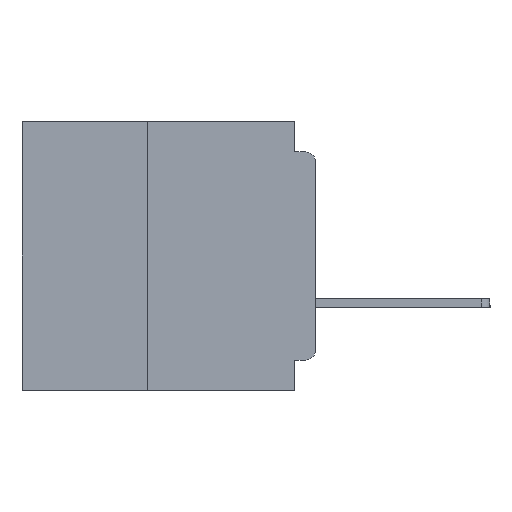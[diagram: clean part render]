
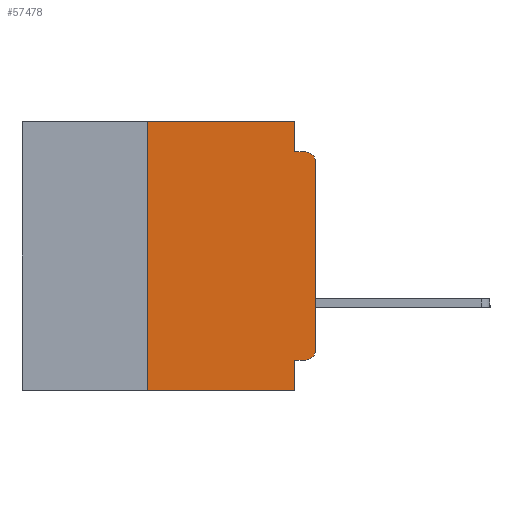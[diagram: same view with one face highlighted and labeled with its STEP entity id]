
A CAD part, left-side view. The second image highlights one B-rep face of the part: STEP entity #57478.
In plain terms, the highlighted planar face has unit normal (-1, 0, 0).
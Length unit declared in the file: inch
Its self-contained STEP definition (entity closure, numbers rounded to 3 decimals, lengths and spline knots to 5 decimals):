
#127 = CARTESIAN_POINT ( 'NONE',  ( 0., 0., 0. ) ) ;
#423 = VERTEX_POINT ( 'NONE', #56707 ) ;
#825 = VECTOR ( 'NONE', #41321, 39.37008 ) ;
#892 = AXIS2_PLACEMENT_3D ( 'NONE', #45539, #17792, #50146 ) ;
#1173 = ORIENTED_EDGE ( 'NONE', *, *, #5365, .F. ) ;
#2561 = CARTESIAN_POINT ( 'NONE',  ( 0., 0., -0.06 ) ) ;
#2929 = DIRECTION ( 'NONE',  ( 0., 1., 0. ) ) ;
#3710 = CARTESIAN_POINT ( 'NONE',  ( 0., 0., -0.045 ) ) ;
#4308 = VECTOR ( 'NONE', #13900, 39.37008 ) ;
#5365 = EDGE_CURVE ( 'NONE', #21179, #18972, #5542, .T. ) ;
#5480 = ORIENTED_EDGE ( 'NONE', *, *, #29334, .T. ) ;
#5542 = LINE ( 'NONE', #45317, #53312 ) ;
#7944 = CARTESIAN_POINT ( 'NONE',  ( 0., 0.015, -0.045 ) ) ;
#8990 = VECTOR ( 'NONE', #28666, 39.37008 ) ;
#9061 = ORIENTED_EDGE ( 'NONE', *, *, #54121, .F. ) ;
#9487 = ORIENTED_EDGE ( 'NONE', *, *, #53385, .T. ) ;
#10893 = VERTEX_POINT ( 'NONE', #15978 ) ;
#11101 = AXIS2_PLACEMENT_3D ( 'NONE', #27559, #59722, #32223 ) ;
#11549 = CARTESIAN_POINT ( 'NONE',  ( 0., 0.031, -0.045 ) ) ;
#12490 = VERTEX_POINT ( 'NONE', #18431 ) ;
#13452 = EDGE_CURVE ( 'NONE', #12490, #41542, #34799, .T. ) ;
#13900 = DIRECTION ( 'NONE',  ( 0., 0., -1. ) ) ;
#15310 = LINE ( 'NONE', #41620, #4308 ) ;
#15370 = VERTEX_POINT ( 'NONE', #2561 ) ;
#15978 = CARTESIAN_POINT ( 'NONE',  ( 0., 0.031, -0.4 ) ) ;
#16665 = VERTEX_POINT ( 'NONE', #7944 ) ;
#16873 = EDGE_CURVE ( 'NONE', #423, #15370, #31400, .T. ) ;
#17481 = DIRECTION ( 'NONE',  ( 0., 0., -1. ) ) ;
#17766 = DIRECTION ( 'NONE',  ( 0., 0., 1. ) ) ;
#17792 = DIRECTION ( 'NONE',  ( -1., 0., 0. ) ) ;
#18021 = DIRECTION ( 'NONE',  ( 0., -1., 0. ) ) ;
#18431 = CARTESIAN_POINT ( 'NONE',  ( 0., 0.031, 0. ) ) ;
#18620 = CARTESIAN_POINT ( 'NONE',  ( 0., 0.015, -0.355 ) ) ;
#18631 = CARTESIAN_POINT ( 'NONE',  ( 0., 0.437, 0. ) ) ;
#18972 = VERTEX_POINT ( 'NONE', #28121 ) ;
#19666 = VERTEX_POINT ( 'NONE', #52303 ) ;
#20979 = AXIS2_PLACEMENT_3D ( 'NONE', #18631, #55702, #28078 ) ;
#21026 = EDGE_CURVE ( 'NONE', #41542, #16665, #30365, .T. ) ;
#21179 = VERTEX_POINT ( 'NONE', #46736 ) ;
#22640 = EDGE_CURVE ( 'NONE', #25651, #19666, #46860, .T. ) ;
#25612 = LINE ( 'NONE', #33304, #8990 ) ;
#25651 = VERTEX_POINT ( 'NONE', #18620 ) ;
#26751 = CARTESIAN_POINT ( 'NONE',  ( 0., 0.031, 0. ) ) ;
#27559 = CARTESIAN_POINT ( 'NONE',  ( 0., 0.015, -0.06 ) ) ;
#27973 = DIRECTION ( 'NONE',  ( 0., 0., 1. ) ) ;
#28078 = DIRECTION ( 'NONE',  ( 0., 0., -1. ) ) ;
#28121 = CARTESIAN_POINT ( 'NONE',  ( 0., 0.25, 0. ) ) ;
#28666 = DIRECTION ( 'NONE',  ( 0., -1., 0. ) ) ;
#29334 = EDGE_CURVE ( 'NONE', #21179, #10893, #25612, .T. ) ;
#30365 = LINE ( 'NONE', #3710, #41311 ) ;
#31400 = LINE ( 'NONE', #127, #54470 ) ;
#32158 = CARTESIAN_POINT ( 'NONE',  ( 0., 0.437, 0. ) ) ;
#32223 = DIRECTION ( 'NONE',  ( 0., 0., -1. ) ) ;
#33004 = ORIENTED_EDGE ( 'NONE', *, *, #16873, .T. ) ;
#33077 = VECTOR ( 'NONE', #2929, 39.37008 ) ;
#33304 = CARTESIAN_POINT ( 'NONE',  ( 0., 0.437, -0.4 ) ) ;
#34318 = ORIENTED_EDGE ( 'NONE', *, *, #58451, .F. ) ;
#34799 = LINE ( 'NONE', #26751, #42806 ) ;
#35270 = ORIENTED_EDGE ( 'NONE', *, *, #13452, .F. ) ;
#41311 = VECTOR ( 'NONE', #18021, 39.37008 ) ;
#41321 = DIRECTION ( 'NONE',  ( 0., -1., 0. ) ) ;
#41542 = VERTEX_POINT ( 'NONE', #11549 ) ;
#41620 = CARTESIAN_POINT ( 'NONE',  ( 0., 0.031, -0.4 ) ) ;
#42573 = EDGE_LOOP ( 'NONE', ( #33004, #50265, #50708, #35270, #34318, #1173, #5480, #9061, #47367, #9487 ) ) ;
#42806 = VECTOR ( 'NONE', #17481, 39.37008 ) ;
#43650 = CIRCLE ( 'NONE', #892, 0.015 ) ;
#44791 = CARTESIAN_POINT ( 'NONE',  ( 0., 0., -0.355 ) ) ;
#45317 = CARTESIAN_POINT ( 'NONE',  ( 0., 0.25, -0.4 ) ) ;
#45539 = CARTESIAN_POINT ( 'NONE',  ( 0., 0.015, -0.34 ) ) ;
#46736 = CARTESIAN_POINT ( 'NONE',  ( 0., 0.25, -0.4 ) ) ;
#46860 = LINE ( 'NONE', #44791, #33077 ) ;
#47367 = ORIENTED_EDGE ( 'NONE', *, *, #22640, .F. ) ;
#49621 = FACE_OUTER_BOUND ( 'NONE', #42573, .T. ) ;
#50146 = DIRECTION ( 'NONE',  ( 0., 0., -1. ) ) ;
#50200 = LINE ( 'NONE', #32158, #825 ) ;
#50265 = ORIENTED_EDGE ( 'NONE', *, *, #51564, .T. ) ;
#50708 = ORIENTED_EDGE ( 'NONE', *, *, #21026, .F. ) ;
#51144 = PLANE ( 'NONE',  #20979 ) ;
#51564 = EDGE_CURVE ( 'NONE', #15370, #16665, #54487, .T. ) ;
#52303 = CARTESIAN_POINT ( 'NONE',  ( 0., 0.031, -0.355 ) ) ;
#53312 = VECTOR ( 'NONE', #17766, 39.37008 ) ;
#53385 = EDGE_CURVE ( 'NONE', #25651, #423, #43650, .T. ) ;
#54121 = EDGE_CURVE ( 'NONE', #19666, #10893, #15310, .T. ) ;
#54470 = VECTOR ( 'NONE', #27973, 39.37008 ) ;
#54487 = CIRCLE ( 'NONE', #11101, 0.015 ) ;
#55702 = DIRECTION ( 'NONE',  ( 1., 0., 0. ) ) ;
#56707 = CARTESIAN_POINT ( 'NONE',  ( 0., 0., -0.34 ) ) ;
#57478 = ADVANCED_FACE ( 'NONE', ( #49621 ), #51144, .F. ) ;
#58451 = EDGE_CURVE ( 'NONE', #18972, #12490, #50200, .T. ) ;
#59722 = DIRECTION ( 'NONE',  ( -1., 0., 0. ) ) ;
